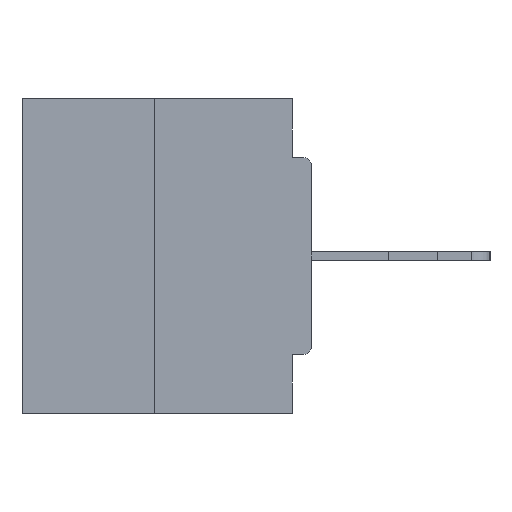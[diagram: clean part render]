
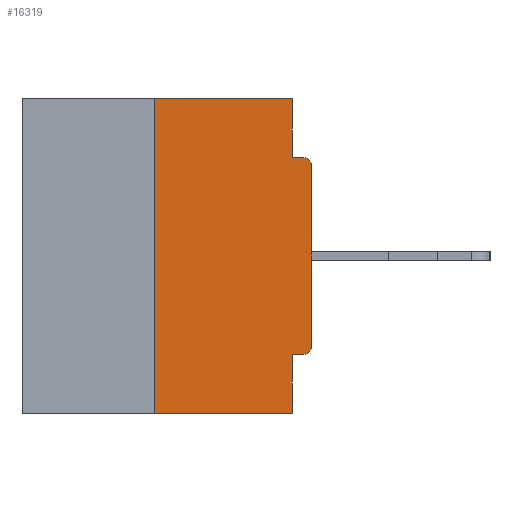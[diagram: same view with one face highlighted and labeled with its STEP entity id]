
A CAD part, left-side view. The second image highlights one B-rep face of the part: STEP entity #16319.
In plain terms, the highlighted planar face has unit normal (-1, 0, 0).
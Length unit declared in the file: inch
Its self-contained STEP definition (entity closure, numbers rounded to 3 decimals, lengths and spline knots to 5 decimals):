
#78 = CARTESIAN_POINT ( 'NONE',  ( 0., 0.031, -0.5 ) ) ;
#329 = CARTESIAN_POINT ( 'NONE',  ( 0., 0.031, 0. ) ) ;
#659 = DIRECTION ( 'NONE',  ( 0., -1., 0. ) ) ;
#807 = LINE ( 'NONE', #23199, #23535 ) ;
#1064 = VERTEX_POINT ( 'NONE', #17530 ) ;
#1144 = EDGE_CURVE ( 'NONE', #4153, #1064, #24180, .T. ) ;
#1509 = VERTEX_POINT ( 'NONE', #27220 ) ;
#1662 = DIRECTION ( 'NONE',  ( 0., 0., -1. ) ) ;
#1670 = LINE ( 'NONE', #10727, #24081 ) ;
#1811 = AXIS2_PLACEMENT_3D ( 'NONE', #2694, #18121, #15891 ) ;
#2228 = CARTESIAN_POINT ( 'NONE',  ( 0., 0., -0.4065 ) ) ;
#2288 = EDGE_CURVE ( 'NONE', #29015, #10462, #21314, .T. ) ;
#2465 = CARTESIAN_POINT ( 'NONE',  ( 0., 0.031, -0.4065 ) ) ;
#2469 = VECTOR ( 'NONE', #6027, 39.37008 ) ;
#2694 = CARTESIAN_POINT ( 'NONE',  ( 0., 0.46, 0. ) ) ;
#3472 = ORIENTED_EDGE ( 'NONE', *, *, #14303, .F. ) ;
#3891 = CARTESIAN_POINT ( 'NONE',  ( 0., 0.25, 0. ) ) ;
#4093 = CARTESIAN_POINT ( 'NONE',  ( 0., 0.015, -0.0935 ) ) ;
#4153 = VERTEX_POINT ( 'NONE', #15338 ) ;
#4331 = DIRECTION ( 'NONE',  ( 0., 0., 1. ) ) ;
#4642 = DIRECTION ( 'NONE',  ( -1., 0., 0. ) ) ;
#4889 = CIRCLE ( 'NONE', #8672, 0.015 ) ;
#5002 = ORIENTED_EDGE ( 'NONE', *, *, #13080, .F. ) ;
#5216 = AXIS2_PLACEMENT_3D ( 'NONE', #22110, #21966, #1662 ) ;
#5558 = VECTOR ( 'NONE', #25277, 39.37008 ) ;
#6027 = DIRECTION ( 'NONE',  ( 0., 0., -1. ) ) ;
#6570 = CARTESIAN_POINT ( 'NONE',  ( 0., 0., -0.1085 ) ) ;
#6638 = ORIENTED_EDGE ( 'NONE', *, *, #15685, .F. ) ;
#6854 = PLANE ( 'NONE',  #1811 ) ;
#7058 = LINE ( 'NONE', #15800, #15562 ) ;
#7121 = VERTEX_POINT ( 'NONE', #6570 ) ;
#7282 = EDGE_CURVE ( 'NONE', #7121, #20223, #4889, .T. ) ;
#8387 = EDGE_CURVE ( 'NONE', #29015, #26955, #25332, .T. ) ;
#8672 = AXIS2_PLACEMENT_3D ( 'NONE', #20494, #4642, #11601 ) ;
#8834 = CARTESIAN_POINT ( 'NONE',  ( 0., 0., -0.3915 ) ) ;
#9078 = FACE_OUTER_BOUND ( 'NONE', #19284, .T. ) ;
#9387 = CARTESIAN_POINT ( 'NONE',  ( 0., 0.031, 0. ) ) ;
#10462 = VERTEX_POINT ( 'NONE', #8834 ) ;
#10727 = CARTESIAN_POINT ( 'NONE',  ( 0., 0.46, -0.5 ) ) ;
#11601 = DIRECTION ( 'NONE',  ( 0., 0., -1. ) ) ;
#12488 = VERTEX_POINT ( 'NONE', #19548 ) ;
#12870 = ORIENTED_EDGE ( 'NONE', *, *, #1144, .F. ) ;
#13080 = EDGE_CURVE ( 'NONE', #1509, #20223, #7058, .T. ) ;
#13832 = LINE ( 'NONE', #329, #2469 ) ;
#14303 = EDGE_CURVE ( 'NONE', #26955, #12488, #20687, .T. ) ;
#14652 = ORIENTED_EDGE ( 'NONE', *, *, #17392, .T. ) ;
#15338 = CARTESIAN_POINT ( 'NONE',  ( 0., 0.25, -0.5 ) ) ;
#15562 = VECTOR ( 'NONE', #22309, 39.37008 ) ;
#15685 = EDGE_CURVE ( 'NONE', #1064, #24396, #807, .T. ) ;
#15800 = CARTESIAN_POINT ( 'NONE',  ( 0., 0., -0.0935 ) ) ;
#15891 = DIRECTION ( 'NONE',  ( 0., 0., -1. ) ) ;
#15995 = VECTOR ( 'NONE', #4331, 39.37008 ) ;
#16319 = ADVANCED_FACE ( 'NONE', ( #9078 ), #6854, .F. ) ;
#17227 = ORIENTED_EDGE ( 'NONE', *, *, #7282, .T. ) ;
#17392 = EDGE_CURVE ( 'NONE', #4153, #12488, #1670, .T. ) ;
#17530 = CARTESIAN_POINT ( 'NONE',  ( 0., 0.25, 0. ) ) ;
#18121 = DIRECTION ( 'NONE',  ( 1., 0., 0. ) ) ;
#19284 = EDGE_LOOP ( 'NONE', ( #6638, #12870, #14652, #3472, #22812, #27123, #28184, #17227, #5002, #21321 ) ) ;
#19548 = CARTESIAN_POINT ( 'NONE',  ( 0., 0.031, -0.5 ) ) ;
#20223 = VERTEX_POINT ( 'NONE', #4093 ) ;
#20307 = DIRECTION ( 'NONE',  ( 0., 1., 0. ) ) ;
#20494 = CARTESIAN_POINT ( 'NONE',  ( 0., 0.015, -0.1085 ) ) ;
#20687 = LINE ( 'NONE', #78, #5558 ) ;
#21314 = CIRCLE ( 'NONE', #5216, 0.015 ) ;
#21321 = ORIENTED_EDGE ( 'NONE', *, *, #22143, .F. ) ;
#21966 = DIRECTION ( 'NONE',  ( -1., 0., 0. ) ) ;
#22110 = CARTESIAN_POINT ( 'NONE',  ( 0., 0.015, -0.3915 ) ) ;
#22143 = EDGE_CURVE ( 'NONE', #24396, #1509, #13832, .T. ) ;
#22309 = DIRECTION ( 'NONE',  ( 0., -1., 0. ) ) ;
#22812 = ORIENTED_EDGE ( 'NONE', *, *, #8387, .F. ) ;
#23199 = CARTESIAN_POINT ( 'NONE',  ( 0., 0.46, 0. ) ) ;
#23535 = VECTOR ( 'NONE', #659, 39.37008 ) ;
#24081 = VECTOR ( 'NONE', #29249, 39.37008 ) ;
#24180 = LINE ( 'NONE', #3891, #15995 ) ;
#24396 = VERTEX_POINT ( 'NONE', #9387 ) ;
#24402 = VECTOR ( 'NONE', #20307, 39.37008 ) ;
#24623 = DIRECTION ( 'NONE',  ( 0., 0., 1. ) ) ;
#25277 = DIRECTION ( 'NONE',  ( 0., 0., -1. ) ) ;
#25332 = LINE ( 'NONE', #2228, #24402 ) ;
#25894 = EDGE_CURVE ( 'NONE', #10462, #7121, #29082, .T. ) ;
#26955 = VERTEX_POINT ( 'NONE', #2465 ) ;
#27123 = ORIENTED_EDGE ( 'NONE', *, *, #2288, .T. ) ;
#27220 = CARTESIAN_POINT ( 'NONE',  ( 0., 0.031, -0.0935 ) ) ;
#28184 = ORIENTED_EDGE ( 'NONE', *, *, #25894, .T. ) ;
#28479 = CARTESIAN_POINT ( 'NONE',  ( 0., 0., 0. ) ) ;
#28554 = VECTOR ( 'NONE', #24623, 39.37008 ) ;
#29015 = VERTEX_POINT ( 'NONE', #29123 ) ;
#29082 = LINE ( 'NONE', #28479, #28554 ) ;
#29123 = CARTESIAN_POINT ( 'NONE',  ( 0., 0.015, -0.4065 ) ) ;
#29249 = DIRECTION ( 'NONE',  ( 0., -1., 0. ) ) ;
